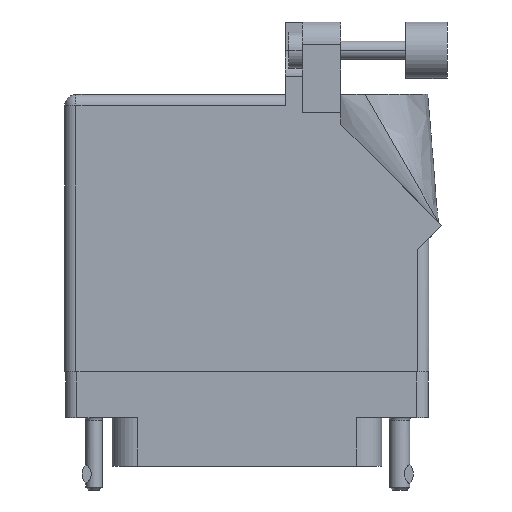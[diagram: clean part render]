
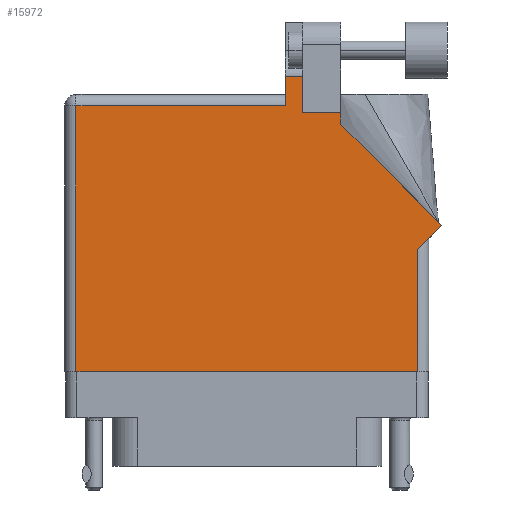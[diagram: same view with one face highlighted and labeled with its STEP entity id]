
A CAD part, front view. The second image highlights one B-rep face of the part: STEP entity #15972.
In plain terms, the highlighted face is planar.
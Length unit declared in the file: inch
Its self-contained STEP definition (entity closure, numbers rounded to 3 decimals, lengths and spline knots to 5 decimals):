
#875 = DIRECTION ( 'NONE',  ( 0., 0., -1. ) ) ;
#1786 = LINE ( 'NONE', #34602, #13177 ) ;
#2011 = DIRECTION ( 'NONE',  ( 0., 1., 0. ) ) ;
#2976 = CARTESIAN_POINT ( 'NONE',  ( -0.943, 1.368, 0.455 ) ) ;
#3757 = CARTESIAN_POINT ( 'NONE',  ( -1.005, -0.1, 0.455 ) ) ;
#5097 = VERTEX_POINT ( 'NONE', #19582 ) ;
#5468 = VECTOR ( 'NONE', #2011, 39.37008 ) ;
#5555 = EDGE_CURVE ( 'NONE', #9109, #5097, #22781, .T. ) ;
#5850 = LINE ( 'NONE', #46107, #44778 ) ;
#6180 = DIRECTION ( 'NONE',  ( -0.707, 0.707, 0. ) ) ;
#6678 = CARTESIAN_POINT ( 'NONE',  ( 1.07571, 0.70771, 0.455 ) ) ;
#7208 = VECTOR ( 'NONE', #28136, 39.37008 ) ;
#7950 = DIRECTION ( 'NONE',  ( 1., 0., 0. ) ) ;
#8226 = LINE ( 'NONE', #3757, #47761 ) ;
#8283 = VERTEX_POINT ( 'NONE', #48107 ) ;
#9064 = LINE ( 'NONE', #39162, #22215 ) ;
#9109 = VERTEX_POINT ( 'NONE', #49205 ) ;
#9462 = ORIENTED_EDGE ( 'NONE', *, *, #48286, .T. ) ;
#9795 = VECTOR ( 'NONE', #22754, 39.37008 ) ;
#10439 = EDGE_CURVE ( 'NONE', #8283, #29987, #9064, .T. ) ;
#10515 = EDGE_CURVE ( 'NONE', #30963, #18421, #19770, .T. ) ;
#10746 = EDGE_CURVE ( 'NONE', #22886, #9109, #37778, .T. ) ;
#10836 = VECTOR ( 'NONE', #46052, 39.37008 ) ;
#11135 = DIRECTION ( 'NONE',  ( -1., 0., 0. ) ) ;
#12238 = ORIENTED_EDGE ( 'NONE', *, *, #10515, .T. ) ;
#12773 = EDGE_CURVE ( 'NONE', #32789, #34620, #29201, .T. ) ;
#12837 = ORIENTED_EDGE ( 'NONE', *, *, #26143, .T. ) ;
#12947 = CARTESIAN_POINT ( 'NONE',  ( -1.005, 1.43, 0.455 ) ) ;
#13177 = VECTOR ( 'NONE', #27047, 39.37008 ) ;
#15163 = ORIENTED_EDGE ( 'NONE', *, *, #12773, .T. ) ;
#15332 = ORIENTED_EDGE ( 'NONE', *, *, #17677, .T. ) ;
#15972 = ADVANCED_FACE ( 'NONE', ( #17594 ), #38237, .F. ) ;
#16123 = CARTESIAN_POINT ( 'NONE',  ( 0.519, 1.26442, 0.455 ) ) ;
#16153 = LINE ( 'NONE', #27642, #7208 ) ;
#16200 = CARTESIAN_POINT ( 'NONE',  ( 0.519, 1.33, 0.455 ) ) ;
#16231 = AXIS2_PLACEMENT_3D ( 'NONE', #12947, #875, #19950 ) ;
#17594 = FACE_OUTER_BOUND ( 'NONE', #29583, .T. ) ;
#17677 = EDGE_CURVE ( 'NONE', #29987, #32789, #34859, .T. ) ;
#18144 = ORIENTED_EDGE ( 'NONE', *, *, #10746, .T. ) ;
#18421 = VERTEX_POINT ( 'NONE', #44071 ) ;
#19230 = CARTESIAN_POINT ( 'NONE',  ( -0.943, -0.1, 0.455 ) ) ;
#19582 = CARTESIAN_POINT ( 'NONE',  ( 0.212, 1.5315, 0.455 ) ) ;
#19770 = LINE ( 'NONE', #19230, #10836 ) ;
#19832 = VECTOR ( 'NONE', #6180, 39.37008 ) ;
#19950 = DIRECTION ( 'NONE',  ( -1., 0., 0. ) ) ;
#20186 = ORIENTED_EDGE ( 'NONE', *, *, #45425, .T. ) ;
#21575 = CARTESIAN_POINT ( 'NONE',  ( 0.212, 1.368, 0.455 ) ) ;
#22215 = VECTOR ( 'NONE', #30814, 39.37008 ) ;
#22754 = DIRECTION ( 'NONE',  ( -1., 0., 0. ) ) ;
#22781 = LINE ( 'NONE', #42312, #44363 ) ;
#22886 = VERTEX_POINT ( 'NONE', #39927 ) ;
#24355 = EDGE_CURVE ( 'NONE', #27334, #8283, #1786, .T. ) ;
#25081 = DIRECTION ( 'NONE',  ( 0., 1., 0. ) ) ;
#26143 = EDGE_CURVE ( 'NONE', #42431, #30963, #5850, .T. ) ;
#26178 = EDGE_CURVE ( 'NONE', #18421, #27334, #8226, .T. ) ;
#27047 = DIRECTION ( 'NONE',  ( 0., 1., 0. ) ) ;
#27334 = VERTEX_POINT ( 'NONE', #28882 ) ;
#27493 = ORIENTED_EDGE ( 'NONE', *, *, #10439, .T. ) ;
#27642 = CARTESIAN_POINT ( 'NONE',  ( 0.212, 1.43, 0.455 ) ) ;
#28136 = DIRECTION ( 'NONE',  ( 0., -1., 0. ) ) ;
#28882 = CARTESIAN_POINT ( 'NONE',  ( 0.943, -0.1, 0.455 ) ) ;
#29201 = LINE ( 'NONE', #46857, #33415 ) ;
#29583 = EDGE_LOOP ( 'NONE', ( #18144, #40061, #9462, #12837, #12238, #48395, #32620, #27493, #15332, #15163, #20186 ) ) ;
#29987 = VERTEX_POINT ( 'NONE', #41078 ) ;
#30814 = DIRECTION ( 'NONE',  ( 0.707, 0.707, 0. ) ) ;
#30963 = VERTEX_POINT ( 'NONE', #2976 ) ;
#32620 = ORIENTED_EDGE ( 'NONE', *, *, #24355, .T. ) ;
#32789 = VERTEX_POINT ( 'NONE', #16123 ) ;
#33415 = VECTOR ( 'NONE', #25081, 39.37008 ) ;
#33984 = CARTESIAN_POINT ( 'NONE',  ( 0.519, 1.33, 0.455 ) ) ;
#34602 = CARTESIAN_POINT ( 'NONE',  ( 0.943, 0.637, 0.455 ) ) ;
#34620 = VERTEX_POINT ( 'NONE', #16200 ) ;
#34859 = LINE ( 'NONE', #6678, #19832 ) ;
#37778 = LINE ( 'NONE', #40000, #5468 ) ;
#38237 = PLANE ( 'NONE',  #16231 ) ;
#39162 = CARTESIAN_POINT ( 'NONE',  ( 1.005, 0.637, 0.455 ) ) ;
#39927 = CARTESIAN_POINT ( 'NONE',  ( 0.306, 1.33, 0.455 ) ) ;
#40000 = CARTESIAN_POINT ( 'NONE',  ( 0.306, 1.33, 0.455 ) ) ;
#40061 = ORIENTED_EDGE ( 'NONE', *, *, #5555, .T. ) ;
#41078 = CARTESIAN_POINT ( 'NONE',  ( 1.07571, 0.70771, 0.455 ) ) ;
#42312 = CARTESIAN_POINT ( 'NONE',  ( 0.63677, 1.5315, 0.455 ) ) ;
#42431 = VERTEX_POINT ( 'NONE', #21575 ) ;
#42481 = DIRECTION ( 'NONE',  ( -1., 0., 0. ) ) ;
#44071 = CARTESIAN_POINT ( 'NONE',  ( -0.943, -0.1, 0.455 ) ) ;
#44363 = VECTOR ( 'NONE', #42481, 39.37008 ) ;
#44778 = VECTOR ( 'NONE', #11135, 39.37008 ) ;
#45425 = EDGE_CURVE ( 'NONE', #34620, #22886, #49302, .T. ) ;
#46052 = DIRECTION ( 'NONE',  ( 0., -1., 0. ) ) ;
#46107 = CARTESIAN_POINT ( 'NONE',  ( -1.005, 1.368, 0.455 ) ) ;
#46857 = CARTESIAN_POINT ( 'NONE',  ( 0.519, 1.26442, 0.455 ) ) ;
#47761 = VECTOR ( 'NONE', #7950, 39.37008 ) ;
#48107 = CARTESIAN_POINT ( 'NONE',  ( 0.943, 0.575, 0.455 ) ) ;
#48286 = EDGE_CURVE ( 'NONE', #5097, #42431, #16153, .T. ) ;
#48395 = ORIENTED_EDGE ( 'NONE', *, *, #26178, .T. ) ;
#49205 = CARTESIAN_POINT ( 'NONE',  ( 0.306, 1.5315, 0.455 ) ) ;
#49302 = LINE ( 'NONE', #33984, #9795 ) ;
